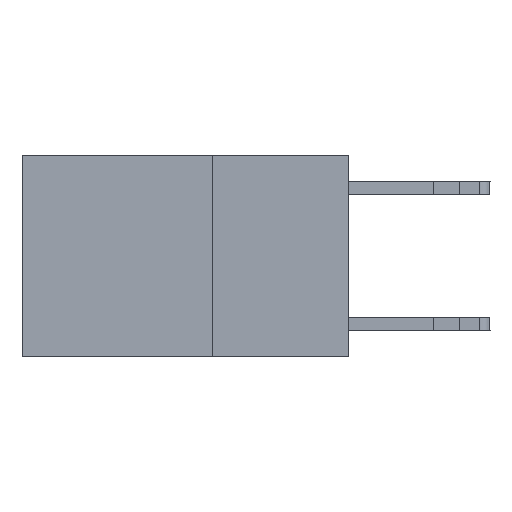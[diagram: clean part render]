
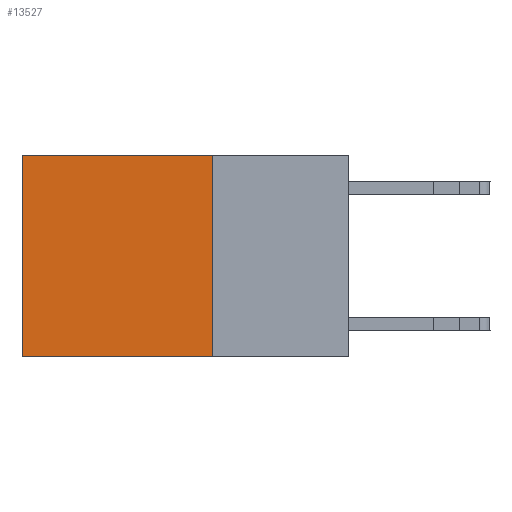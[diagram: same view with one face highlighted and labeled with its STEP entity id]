
A CAD part, left-side view. The second image highlights one B-rep face of the part: STEP entity #13527.
In plain terms, the highlighted planar face has unit normal (-1, 0, 0).
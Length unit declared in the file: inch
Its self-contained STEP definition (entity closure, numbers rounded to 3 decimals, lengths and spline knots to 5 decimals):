
#122 = LINE ( 'NONE', #7129, #13005 ) ;
#1182 = ORIENTED_EDGE ( 'NONE', *, *, #8134, .T. ) ;
#1446 = DIRECTION ( 'NONE',  ( 1., 0., 0. ) ) ;
#1723 = VERTEX_POINT ( 'NONE', #9913 ) ;
#2519 = DIRECTION ( 'NONE',  ( 0., 0., -1. ) ) ;
#3919 = ORIENTED_EDGE ( 'NONE', *, *, #9727, .F. ) ;
#4109 = CARTESIAN_POINT ( 'NONE',  ( 0.2625, 0.25, -0.37 ) ) ;
#4321 = LINE ( 'NONE', #7120, #17037 ) ;
#4435 = DIRECTION ( 'NONE',  ( 0., 0., -1. ) ) ;
#4584 = CARTESIAN_POINT ( 'NONE',  ( 0.2625, 0.6, -0.37 ) ) ;
#5252 = DIRECTION ( 'NONE',  ( 0., 1., 0. ) ) ;
#5498 = CARTESIAN_POINT ( 'NONE',  ( 0.2625, 0.25, 0. ) ) ;
#6021 = EDGE_LOOP ( 'NONE', ( #1182, #3919, #13080, #14765 ) ) ;
#7046 = FACE_OUTER_BOUND ( 'NONE', #6021, .T. ) ;
#7120 = CARTESIAN_POINT ( 'NONE',  ( 0.2625, 0.6, 0. ) ) ;
#7129 = CARTESIAN_POINT ( 'NONE',  ( 0.2625, 0.25, 0. ) ) ;
#7306 = EDGE_CURVE ( 'NONE', #14459, #1723, #12556, .T. ) ;
#7648 = EDGE_CURVE ( 'NONE', #14459, #18313, #122, .T. ) ;
#8134 = EDGE_CURVE ( 'NONE', #1723, #11117, #4321, .T. ) ;
#8388 = AXIS2_PLACEMENT_3D ( 'NONE', #5498, #1446, #17418 ) ;
#9727 = EDGE_CURVE ( 'NONE', #18313, #11117, #12475, .T. ) ;
#9913 = CARTESIAN_POINT ( 'NONE',  ( 0.2625, 0.6, 0. ) ) ;
#10987 = CARTESIAN_POINT ( 'NONE',  ( 0.2625, 0.25, 0. ) ) ;
#11117 = VERTEX_POINT ( 'NONE', #4584 ) ;
#12475 = LINE ( 'NONE', #12567, #13411 ) ;
#12556 = LINE ( 'NONE', #10987, #16251 ) ;
#12567 = CARTESIAN_POINT ( 'NONE',  ( 0.2625, 0.25, -0.37 ) ) ;
#13005 = VECTOR ( 'NONE', #4435, 39.37008 ) ;
#13080 = ORIENTED_EDGE ( 'NONE', *, *, #7648, .F. ) ;
#13411 = VECTOR ( 'NONE', #5252, 39.37008 ) ;
#13527 = ADVANCED_FACE ( 'NONE', ( #7046 ), #15696, .F. ) ;
#14459 = VERTEX_POINT ( 'NONE', #17518 ) ;
#14765 = ORIENTED_EDGE ( 'NONE', *, *, #7306, .T. ) ;
#15696 = PLANE ( 'NONE',  #8388 ) ;
#16251 = VECTOR ( 'NONE', #18418, 39.37008 ) ;
#17037 = VECTOR ( 'NONE', #2519, 39.37008 ) ;
#17418 = DIRECTION ( 'NONE',  ( 0., 0., -1. ) ) ;
#17518 = CARTESIAN_POINT ( 'NONE',  ( 0.2625, 0.25, 0. ) ) ;
#18313 = VERTEX_POINT ( 'NONE', #4109 ) ;
#18418 = DIRECTION ( 'NONE',  ( 0., 1., 0. ) ) ;
